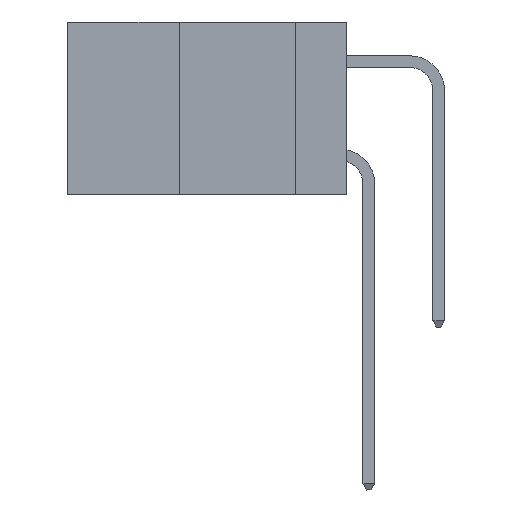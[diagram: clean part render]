
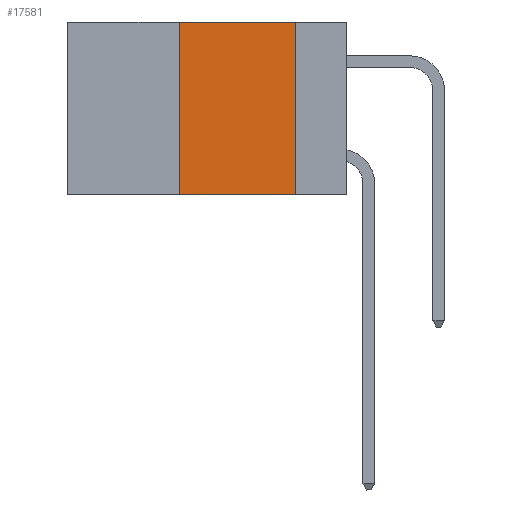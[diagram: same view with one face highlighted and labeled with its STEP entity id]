
A CAD part, left-side view. The second image highlights one B-rep face of the part: STEP entity #17581.
In plain terms, the highlighted planar face has unit normal (-1, 0, 0).
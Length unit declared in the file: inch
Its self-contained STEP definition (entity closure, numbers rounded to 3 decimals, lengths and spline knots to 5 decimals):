
#2174 = VERTEX_POINT ( 'NONE', #4004 ) ;
#2197 = CARTESIAN_POINT ( 'NONE',  ( 0., 0.6, -0.37 ) ) ;
#3315 = VERTEX_POINT ( 'NONE', #9232 ) ;
#3766 = DIRECTION ( 'NONE',  ( 0., 0., -1. ) ) ;
#3922 = EDGE_LOOP ( 'NONE', ( #23453, #4642, #19975, #23211 ) ) ;
#4004 = CARTESIAN_POINT ( 'NONE',  ( 0., 0.11, -0.37 ) ) ;
#4333 = LINE ( 'NONE', #16803, #20218 ) ;
#4642 = ORIENTED_EDGE ( 'NONE', *, *, #13361, .F. ) ;
#4802 = LINE ( 'NONE', #15267, #24528 ) ;
#5301 = DIRECTION ( 'NONE',  ( 0., 0., 1. ) ) ;
#6212 = VECTOR ( 'NONE', #14604, 39.37008 ) ;
#7322 = EDGE_CURVE ( 'NONE', #19567, #2174, #16536, .T. ) ;
#8289 = VERTEX_POINT ( 'NONE', #22247 ) ;
#9232 = CARTESIAN_POINT ( 'NONE',  ( 0., 0.36, 0. ) ) ;
#9309 = DIRECTION ( 'NONE',  ( 1., 0., 0. ) ) ;
#11433 = VECTOR ( 'NONE', #11862, 39.37008 ) ;
#11862 = DIRECTION ( 'NONE',  ( 0., -1., 0. ) ) ;
#11951 = LINE ( 'NONE', #18382, #6212 ) ;
#13113 = CARTESIAN_POINT ( 'NONE',  ( 0., 0.6, 0. ) ) ;
#13361 = EDGE_CURVE ( 'NONE', #3315, #8289, #11951, .T. ) ;
#14604 = DIRECTION ( 'NONE',  ( 0., -1., 0. ) ) ;
#15267 = CARTESIAN_POINT ( 'NONE',  ( 0., 0.11, 0. ) ) ;
#16201 = FACE_OUTER_BOUND ( 'NONE', #3922, .T. ) ;
#16536 = LINE ( 'NONE', #2197, #11433 ) ;
#16803 = CARTESIAN_POINT ( 'NONE',  ( 0., 0.36, 0. ) ) ;
#16940 = PLANE ( 'NONE',  #20128 ) ;
#17581 = ADVANCED_FACE ( 'NONE', ( #16201 ), #16940, .F. ) ;
#17639 = EDGE_CURVE ( 'NONE', #8289, #2174, #4802, .T. ) ;
#18382 = CARTESIAN_POINT ( 'NONE',  ( 0., 0.6, 0. ) ) ;
#19567 = VERTEX_POINT ( 'NONE', #23425 ) ;
#19975 = ORIENTED_EDGE ( 'NONE', *, *, #21783, .F. ) ;
#20128 = AXIS2_PLACEMENT_3D ( 'NONE', #13113, #9309, #22667 ) ;
#20218 = VECTOR ( 'NONE', #5301, 39.37008 ) ;
#21783 = EDGE_CURVE ( 'NONE', #19567, #3315, #4333, .T. ) ;
#22247 = CARTESIAN_POINT ( 'NONE',  ( 0., 0.11, 0. ) ) ;
#22667 = DIRECTION ( 'NONE',  ( 0., 0., -1. ) ) ;
#23211 = ORIENTED_EDGE ( 'NONE', *, *, #7322, .T. ) ;
#23425 = CARTESIAN_POINT ( 'NONE',  ( 0., 0.36, -0.37 ) ) ;
#23453 = ORIENTED_EDGE ( 'NONE', *, *, #17639, .F. ) ;
#24528 = VECTOR ( 'NONE', #3766, 39.37008 ) ;
